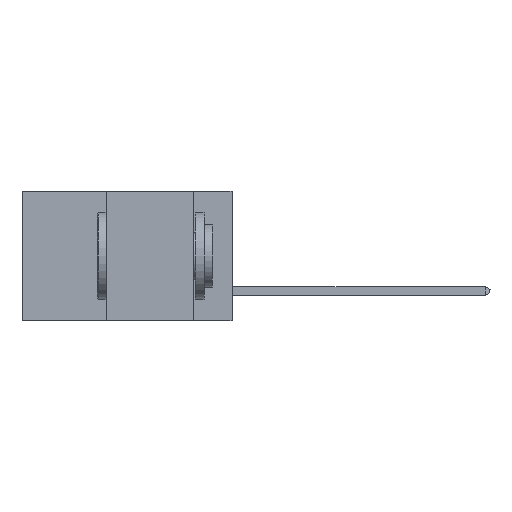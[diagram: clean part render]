
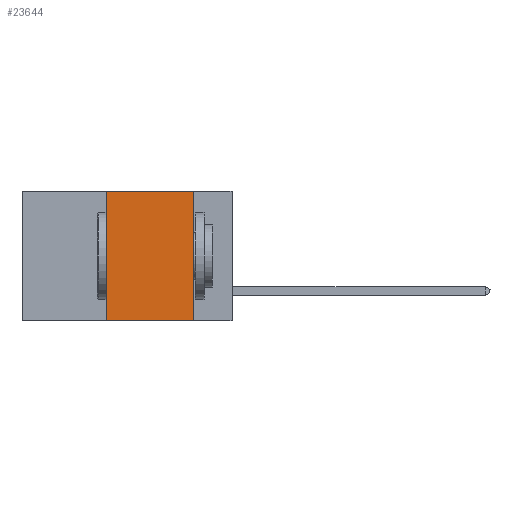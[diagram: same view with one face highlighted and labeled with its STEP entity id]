
A CAD part, left-side view. The second image highlights one B-rep face of the part: STEP entity #23644.
In plain terms, the highlighted planar face has unit normal (-1, 0, 0).
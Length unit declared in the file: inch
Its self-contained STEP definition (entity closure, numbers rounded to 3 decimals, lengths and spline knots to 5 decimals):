
#143 = VERTEX_POINT ( 'NONE', #31249 ) ;
#1321 = VECTOR ( 'NONE', #21120, 39.37008 ) ;
#1419 = CARTESIAN_POINT ( 'NONE',  ( 0., 0.11, 0. ) ) ;
#1975 = EDGE_LOOP ( 'NONE', ( #31895, #24453, #29670, #33022 ) ) ;
#2650 = CARTESIAN_POINT ( 'NONE',  ( 0., 0.6, 0. ) ) ;
#4718 = VERTEX_POINT ( 'NONE', #22372 ) ;
#5448 = VERTEX_POINT ( 'NONE', #26332 ) ;
#7710 = VECTOR ( 'NONE', #25968, 39.37008 ) ;
#8037 = CARTESIAN_POINT ( 'NONE',  ( 0., 0.6, 0. ) ) ;
#11546 = LINE ( 'NONE', #26463, #1321 ) ;
#16538 = EDGE_CURVE ( 'NONE', #143, #5448, #11546, .T. ) ;
#16829 = LINE ( 'NONE', #23182, #28354 ) ;
#18009 = DIRECTION ( 'NONE',  ( 0., 0., 1. ) ) ;
#19964 = VECTOR ( 'NONE', #32927, 39.37008 ) ;
#21120 = DIRECTION ( 'NONE',  ( 0., -1., 0. ) ) ;
#22372 = CARTESIAN_POINT ( 'NONE',  ( 0., 0.36, 0. ) ) ;
#22662 = EDGE_CURVE ( 'NONE', #29722, #5448, #29017, .T. ) ;
#23182 = CARTESIAN_POINT ( 'NONE',  ( 0., 0.36, 0. ) ) ;
#23644 = ADVANCED_FACE ( 'NONE', ( #30672 ), #29393, .F. ) ;
#24168 = CARTESIAN_POINT ( 'NONE',  ( 0., 0.11, 0. ) ) ;
#24453 = ORIENTED_EDGE ( 'NONE', *, *, #33354, .F. ) ;
#25968 = DIRECTION ( 'NONE',  ( 0., 0., -1. ) ) ;
#26332 = CARTESIAN_POINT ( 'NONE',  ( 0., 0.11, -0.37 ) ) ;
#26463 = CARTESIAN_POINT ( 'NONE',  ( 0., 0.6, -0.37 ) ) ;
#27009 = DIRECTION ( 'NONE',  ( 1., 0., 0. ) ) ;
#28246 = EDGE_CURVE ( 'NONE', #143, #4718, #16829, .T. ) ;
#28354 = VECTOR ( 'NONE', #18009, 39.37008 ) ;
#29017 = LINE ( 'NONE', #1419, #7710 ) ;
#29330 = LINE ( 'NONE', #2650, #19964 ) ;
#29393 = PLANE ( 'NONE',  #29713 ) ;
#29670 = ORIENTED_EDGE ( 'NONE', *, *, #28246, .F. ) ;
#29713 = AXIS2_PLACEMENT_3D ( 'NONE', #8037, #27009, #29756 ) ;
#29722 = VERTEX_POINT ( 'NONE', #24168 ) ;
#29756 = DIRECTION ( 'NONE',  ( 0., 0., -1. ) ) ;
#30672 = FACE_OUTER_BOUND ( 'NONE', #1975, .T. ) ;
#31249 = CARTESIAN_POINT ( 'NONE',  ( 0., 0.36, -0.37 ) ) ;
#31895 = ORIENTED_EDGE ( 'NONE', *, *, #22662, .F. ) ;
#32927 = DIRECTION ( 'NONE',  ( 0., -1., 0. ) ) ;
#33022 = ORIENTED_EDGE ( 'NONE', *, *, #16538, .T. ) ;
#33354 = EDGE_CURVE ( 'NONE', #4718, #29722, #29330, .T. ) ;
